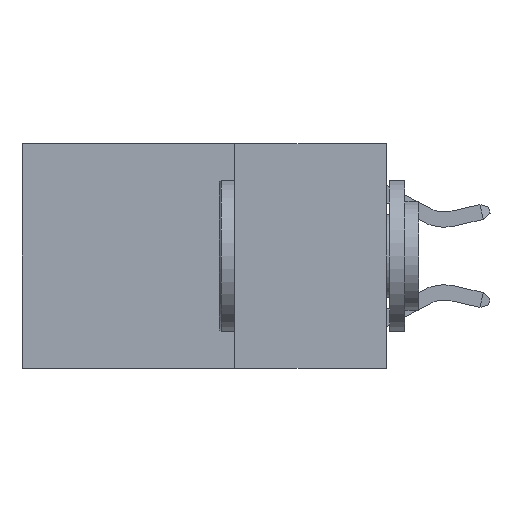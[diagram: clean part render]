
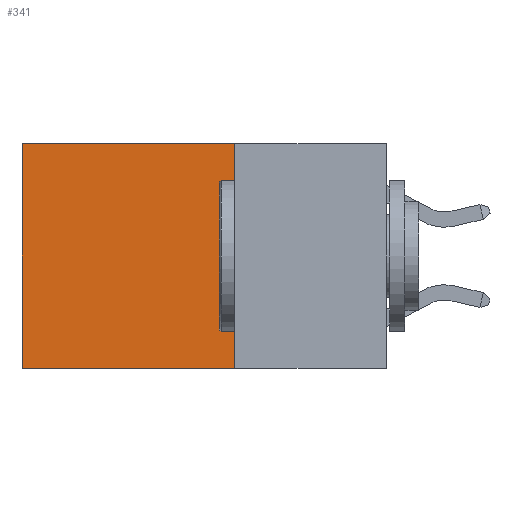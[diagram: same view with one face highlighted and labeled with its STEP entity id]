
A CAD part, left-side view. The second image highlights one B-rep face of the part: STEP entity #341.
In plain terms, the highlighted planar face has unit normal (-1, 0, 0).
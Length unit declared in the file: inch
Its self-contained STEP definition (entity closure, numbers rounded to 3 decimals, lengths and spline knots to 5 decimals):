
#308 = CARTESIAN_POINT ( 'NONE',  ( 0.2625, 0.25, 0. ) ) ;
#341 = ADVANCED_FACE ( 'NONE', ( #6974 ), #11249, .F. ) ;
#1100 = VECTOR ( 'NONE', #7222, 39.37008 ) ;
#1207 = VERTEX_POINT ( 'NONE', #6103 ) ;
#1510 = DIRECTION ( 'NONE',  ( 0., 1., 0. ) ) ;
#1535 = VERTEX_POINT ( 'NONE', #7575 ) ;
#1608 = VERTEX_POINT ( 'NONE', #1827 ) ;
#1694 = ORIENTED_EDGE ( 'NONE', *, *, #2153, .F. ) ;
#1827 = CARTESIAN_POINT ( 'NONE',  ( 0.2625, 0.6, 0. ) ) ;
#2153 = EDGE_CURVE ( 'NONE', #1535, #3935, #10979, .T. ) ;
#2283 = EDGE_LOOP ( 'NONE', ( #4624, #7898, #1694, #11561 ) ) ;
#2856 = EDGE_CURVE ( 'NONE', #3935, #1207, #10770, .T. ) ;
#2979 = CARTESIAN_POINT ( 'NONE',  ( 0.2625, 0.25, 0. ) ) ;
#3015 = DIRECTION ( 'NONE',  ( 0., 0., -1. ) ) ;
#3038 = CARTESIAN_POINT ( 'NONE',  ( 0.2625, 0.25, 0. ) ) ;
#3455 = DIRECTION ( 'NONE',  ( 1., 0., 0. ) ) ;
#3935 = VERTEX_POINT ( 'NONE', #9611 ) ;
#4231 = VECTOR ( 'NONE', #1510, 39.37008 ) ;
#4624 = ORIENTED_EDGE ( 'NONE', *, *, #9526, .T. ) ;
#6103 = CARTESIAN_POINT ( 'NONE',  ( 0.2625, 0.6, -0.37 ) ) ;
#6974 = FACE_OUTER_BOUND ( 'NONE', #2283, .T. ) ;
#7222 = DIRECTION ( 'NONE',  ( 0., 0., -1. ) ) ;
#7575 = CARTESIAN_POINT ( 'NONE',  ( 0.2625, 0.25, 0. ) ) ;
#7898 = ORIENTED_EDGE ( 'NONE', *, *, #2856, .F. ) ;
#8747 = LINE ( 'NONE', #11632, #15188 ) ;
#8953 = CARTESIAN_POINT ( 'NONE',  ( 0.2625, 0.25, -0.37 ) ) ;
#9526 = EDGE_CURVE ( 'NONE', #1608, #1207, #8747, .T. ) ;
#9611 = CARTESIAN_POINT ( 'NONE',  ( 0.2625, 0.25, -0.37 ) ) ;
#9800 = LINE ( 'NONE', #3038, #12666 ) ;
#10405 = DIRECTION ( 'NONE',  ( 0., 1., 0. ) ) ;
#10770 = LINE ( 'NONE', #8953, #4231 ) ;
#10979 = LINE ( 'NONE', #308, #1100 ) ;
#11249 = PLANE ( 'NONE',  #12745 ) ;
#11561 = ORIENTED_EDGE ( 'NONE', *, *, #15214, .T. ) ;
#11632 = CARTESIAN_POINT ( 'NONE',  ( 0.2625, 0.6, 0. ) ) ;
#12666 = VECTOR ( 'NONE', #10405, 39.37008 ) ;
#12745 = AXIS2_PLACEMENT_3D ( 'NONE', #2979, #3455, #14672 ) ;
#14672 = DIRECTION ( 'NONE',  ( 0., 0., -1. ) ) ;
#15188 = VECTOR ( 'NONE', #3015, 39.37008 ) ;
#15214 = EDGE_CURVE ( 'NONE', #1535, #1608, #9800, .T. ) ;
